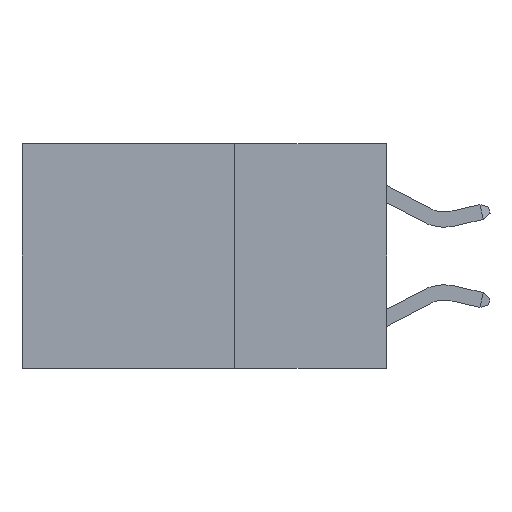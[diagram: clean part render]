
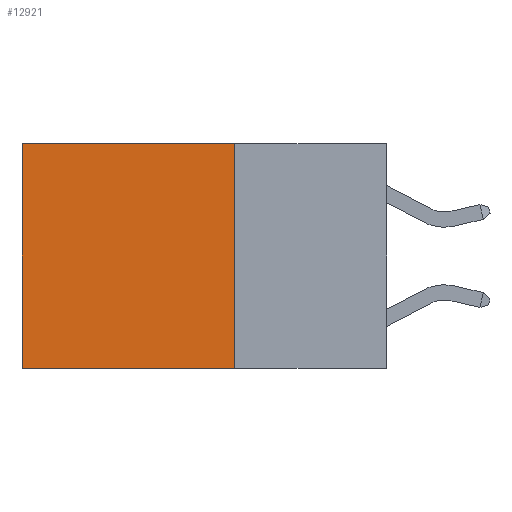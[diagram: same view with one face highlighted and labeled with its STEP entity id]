
A CAD part, left-side view. The second image highlights one B-rep face of the part: STEP entity #12921.
In plain terms, the highlighted planar face has unit normal (-1, 0, 0).
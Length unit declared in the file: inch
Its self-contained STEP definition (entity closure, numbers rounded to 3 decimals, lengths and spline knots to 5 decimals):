
#1196 = CARTESIAN_POINT ( 'NONE',  ( 0.2625, 0.25, 0. ) ) ;
#1936 = LINE ( 'NONE', #8710, #13410 ) ;
#1950 = CARTESIAN_POINT ( 'NONE',  ( 0.2625, 0.6, 0. ) ) ;
#2987 = VECTOR ( 'NONE', #18389, 39.37008 ) ;
#3257 = DIRECTION ( 'NONE',  ( 1., 0., 0. ) ) ;
#4461 = FACE_OUTER_BOUND ( 'NONE', #20815, .T. ) ;
#4492 = EDGE_CURVE ( 'NONE', #23668, #13324, #1936, .T. ) ;
#4547 = EDGE_CURVE ( 'NONE', #20004, #21275, #11830, .T. ) ;
#5210 = PLANE ( 'NONE',  #25885 ) ;
#5362 = CARTESIAN_POINT ( 'NONE',  ( 0.2625, 0.25, 0. ) ) ;
#6698 = VECTOR ( 'NONE', #22146, 39.37008 ) ;
#7362 = CARTESIAN_POINT ( 'NONE',  ( 0.2625, 0.25, 0. ) ) ;
#7538 = ORIENTED_EDGE ( 'NONE', *, *, #4492, .T. ) ;
#7921 = CARTESIAN_POINT ( 'NONE',  ( 0.2625, 0.25, 0. ) ) ;
#8710 = CARTESIAN_POINT ( 'NONE',  ( 0.2625, 0.6, 0. ) ) ;
#9585 = ORIENTED_EDGE ( 'NONE', *, *, #22417, .T. ) ;
#11480 = CARTESIAN_POINT ( 'NONE',  ( 0.2625, 0.6, -0.37 ) ) ;
#11830 = LINE ( 'NONE', #7362, #6698 ) ;
#12068 = VECTOR ( 'NONE', #23826, 39.37008 ) ;
#12921 = ADVANCED_FACE ( 'NONE', ( #4461 ), #5210, .F. ) ;
#12977 = EDGE_CURVE ( 'NONE', #21275, #13324, #20931, .T. ) ;
#13324 = VERTEX_POINT ( 'NONE', #11480 ) ;
#13398 = ORIENTED_EDGE ( 'NONE', *, *, #12977, .F. ) ;
#13410 = VECTOR ( 'NONE', #17878, 39.37008 ) ;
#17820 = CARTESIAN_POINT ( 'NONE',  ( 0.2625, 0.25, -0.37 ) ) ;
#17878 = DIRECTION ( 'NONE',  ( 0., 0., -1. ) ) ;
#18147 = CARTESIAN_POINT ( 'NONE',  ( 0.2625, 0.25, -0.37 ) ) ;
#18389 = DIRECTION ( 'NONE',  ( 0., 1., 0. ) ) ;
#20004 = VERTEX_POINT ( 'NONE', #7921 ) ;
#20815 = EDGE_LOOP ( 'NONE', ( #7538, #13398, #22002, #9585 ) ) ;
#20931 = LINE ( 'NONE', #18147, #12068 ) ;
#21275 = VERTEX_POINT ( 'NONE', #17820 ) ;
#22002 = ORIENTED_EDGE ( 'NONE', *, *, #4547, .F. ) ;
#22146 = DIRECTION ( 'NONE',  ( 0., 0., -1. ) ) ;
#22417 = EDGE_CURVE ( 'NONE', #20004, #23668, #23660, .T. ) ;
#23660 = LINE ( 'NONE', #5362, #2987 ) ;
#23668 = VERTEX_POINT ( 'NONE', #1950 ) ;
#23826 = DIRECTION ( 'NONE',  ( 0., 1., 0. ) ) ;
#25606 = DIRECTION ( 'NONE',  ( 0., 0., -1. ) ) ;
#25885 = AXIS2_PLACEMENT_3D ( 'NONE', #1196, #3257, #25606 ) ;
